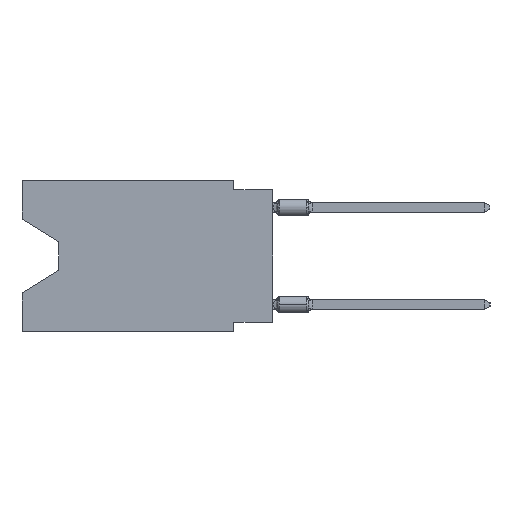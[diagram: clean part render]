
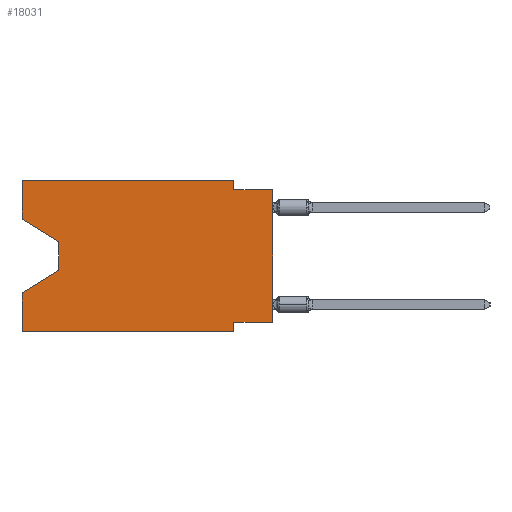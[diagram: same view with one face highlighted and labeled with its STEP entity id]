
A CAD part, left-side view. The second image highlights one B-rep face of the part: STEP entity #18031.
In plain terms, the highlighted planar face has unit normal (-1, 0, 0).
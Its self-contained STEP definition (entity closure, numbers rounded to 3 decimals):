
#53 = LINE ( 'NONE', #33759, #25097 ) ;
#741 = CARTESIAN_POINT ( 'NONE',  ( 0., 13.97, -5.893 ) ) ;
#848 = PLANE ( 'NONE',  #7714 ) ;
#1404 = EDGE_CURVE ( 'NONE', #9565, #9427, #14695, .T. ) ;
#1419 = VECTOR ( 'NONE', #7688, 1000. ) ;
#1522 = LINE ( 'NONE', #12523, #10236 ) ;
#2156 = CARTESIAN_POINT ( 'NONE',  ( 0., 16.383, -9.906 ) ) ;
#2433 = VECTOR ( 'NONE', #32776, 1000. ) ;
#2968 = VECTOR ( 'NONE', #32285, 1000. ) ;
#3423 = VERTEX_POINT ( 'NONE', #2156 ) ;
#4896 = VERTEX_POINT ( 'NONE', #17792 ) ;
#5262 = VECTOR ( 'NONE', #19988, 1000. ) ;
#5466 = CARTESIAN_POINT ( 'NONE',  ( 0., 2.54, -9.906 ) ) ;
#5565 = ORIENTED_EDGE ( 'NONE', *, *, #28004, .F. ) ;
#6286 = CARTESIAN_POINT ( 'NONE',  ( 0., 16.383, 0. ) ) ;
#6357 = ORIENTED_EDGE ( 'NONE', *, *, #11316, .T. ) ;
#6408 = VERTEX_POINT ( 'NONE', #21735 ) ;
#6618 = CARTESIAN_POINT ( 'NONE',  ( 0., 0., 0. ) ) ;
#6856 = VECTOR ( 'NONE', #31949, 1000. ) ;
#7027 = EDGE_CURVE ( 'NONE', #28562, #19460, #29848, .T. ) ;
#7688 = DIRECTION ( 'NONE',  ( 0., 0.855, -0.519 ) ) ;
#7714 = AXIS2_PLACEMENT_3D ( 'NONE', #21823, #32484, #32651 ) ;
#7912 = ORIENTED_EDGE ( 'NONE', *, *, #26705, .F. ) ;
#8039 = LINE ( 'NONE', #26431, #1419 ) ;
#8092 = EDGE_CURVE ( 'NONE', #6408, #10338, #29699, .T. ) ;
#8409 = FACE_OUTER_BOUND ( 'NONE', #16510, .T. ) ;
#8622 = CARTESIAN_POINT ( 'NONE',  ( 0., 16.383, 0. ) ) ;
#8834 = ORIENTED_EDGE ( 'NONE', *, *, #12111, .T. ) ;
#9427 = VERTEX_POINT ( 'NONE', #741 ) ;
#9565 = VERTEX_POINT ( 'NONE', #30663 ) ;
#9892 = CARTESIAN_POINT ( 'NONE',  ( 0., 16.383, -7.36 ) ) ;
#10169 = CARTESIAN_POINT ( 'NONE',  ( 0., 16.383, -9.906 ) ) ;
#10236 = VECTOR ( 'NONE', #30235, 1000. ) ;
#10338 = VERTEX_POINT ( 'NONE', #20717 ) ;
#10534 = DIRECTION ( 'NONE',  ( 0., 0., -1. ) ) ;
#11316 = EDGE_CURVE ( 'NONE', #3423, #22837, #25478, .T. ) ;
#11670 = ORIENTED_EDGE ( 'NONE', *, *, #33593, .F. ) ;
#12111 = EDGE_CURVE ( 'NONE', #16937, #10338, #19340, .T. ) ;
#12229 = ORIENTED_EDGE ( 'NONE', *, *, #7027, .F. ) ;
#12523 = CARTESIAN_POINT ( 'NONE',  ( 0., 16.383, 0. ) ) ;
#12594 = DIRECTION ( 'NONE',  ( 0., -1., 0. ) ) ;
#12970 = VECTOR ( 'NONE', #16502, 1000. ) ;
#13627 = DIRECTION ( 'NONE',  ( 0., 0., 1. ) ) ;
#14222 = LINE ( 'NONE', #29541, #2968 ) ;
#14631 = ORIENTED_EDGE ( 'NONE', *, *, #22446, .F. ) ;
#14695 = LINE ( 'NONE', #30330, #5262 ) ;
#15049 = VECTOR ( 'NONE', #12594, 1000. ) ;
#15448 = EDGE_CURVE ( 'NONE', #9427, #33056, #8039, .T. ) ;
#15841 = ORIENTED_EDGE ( 'NONE', *, *, #32622, .F. ) ;
#16502 = DIRECTION ( 'NONE',  ( 0., 1., 0. ) ) ;
#16510 = EDGE_LOOP ( 'NONE', ( #23887, #22128, #31767, #15841, #6357, #7912, #14631, #8834, #24074, #11670, #12229, #5565 ) ) ;
#16937 = VERTEX_POINT ( 'NONE', #25887 ) ;
#17792 = CARTESIAN_POINT ( 'NONE',  ( 0., 2.54, -9.271 ) ) ;
#18031 = ADVANCED_FACE ( 'NONE', ( #8409 ), #848, .F. ) ;
#18089 = VERTEX_POINT ( 'NONE', #29902 ) ;
#19340 = LINE ( 'NONE', #6618, #2433 ) ;
#19460 = VERTEX_POINT ( 'NONE', #20680 ) ;
#19988 = DIRECTION ( 'NONE',  ( 0., 0., -1. ) ) ;
#20680 = CARTESIAN_POINT ( 'NONE',  ( 0., 2.54, 0. ) ) ;
#20717 = CARTESIAN_POINT ( 'NONE',  ( 0., 0., -0.635 ) ) ;
#21065 = VECTOR ( 'NONE', #13627, 1000. ) ;
#21281 = CARTESIAN_POINT ( 'NONE',  ( 0., 0., -0.635 ) ) ;
#21349 = LINE ( 'NONE', #8622, #21065 ) ;
#21735 = CARTESIAN_POINT ( 'NONE',  ( 0., 2.54, -0.635 ) ) ;
#21823 = CARTESIAN_POINT ( 'NONE',  ( 0., 16.383, 0. ) ) ;
#22128 = ORIENTED_EDGE ( 'NONE', *, *, #1404, .T. ) ;
#22446 = EDGE_CURVE ( 'NONE', #16937, #4896, #31992, .T. ) ;
#22707 = DIRECTION ( 'NONE',  ( 0., 0., -1. ) ) ;
#22837 = VERTEX_POINT ( 'NONE', #5466 ) ;
#23887 = ORIENTED_EDGE ( 'NONE', *, *, #30106, .T. ) ;
#24074 = ORIENTED_EDGE ( 'NONE', *, *, #8092, .F. ) ;
#24728 = CARTESIAN_POINT ( 'NONE',  ( 0., 16.383, 0. ) ) ;
#25097 = VECTOR ( 'NONE', #10534, 1000. ) ;
#25478 = LINE ( 'NONE', #10169, #15049 ) ;
#25887 = CARTESIAN_POINT ( 'NONE',  ( 0., 0., -9.271 ) ) ;
#26077 = VECTOR ( 'NONE', #22707, 1000. ) ;
#26431 = CARTESIAN_POINT ( 'NONE',  ( 0., 13.97, -5.893 ) ) ;
#26705 = EDGE_CURVE ( 'NONE', #4896, #22837, #28432, .T. ) ;
#26842 = CARTESIAN_POINT ( 'NONE',  ( 0., 0., -9.271 ) ) ;
#27913 = CARTESIAN_POINT ( 'NONE',  ( 0., 2.54, -9.906 ) ) ;
#28004 = EDGE_CURVE ( 'NONE', #18089, #28562, #21349, .T. ) ;
#28432 = LINE ( 'NONE', #27913, #26077 ) ;
#28562 = VERTEX_POINT ( 'NONE', #24728 ) ;
#29541 = CARTESIAN_POINT ( 'NONE',  ( 0., 16.383, -2.546 ) ) ;
#29699 = LINE ( 'NONE', #21281, #6856 ) ;
#29848 = LINE ( 'NONE', #6286, #31558 ) ;
#29902 = CARTESIAN_POINT ( 'NONE',  ( 0., 16.383, -2.546 ) ) ;
#30106 = EDGE_CURVE ( 'NONE', #18089, #9565, #14222, .T. ) ;
#30235 = DIRECTION ( 'NONE',  ( 0., 0., 1. ) ) ;
#30330 = CARTESIAN_POINT ( 'NONE',  ( 0., 13.97, -4.013 ) ) ;
#30663 = CARTESIAN_POINT ( 'NONE',  ( 0., 13.97, -4.013 ) ) ;
#31558 = VECTOR ( 'NONE', #32600, 1000. ) ;
#31767 = ORIENTED_EDGE ( 'NONE', *, *, #15448, .T. ) ;
#31949 = DIRECTION ( 'NONE',  ( 0., -1., 0. ) ) ;
#31992 = LINE ( 'NONE', #26842, #12970 ) ;
#32285 = DIRECTION ( 'NONE',  ( 0., -0.855, -0.519 ) ) ;
#32484 = DIRECTION ( 'NONE',  ( 1., 0., 0. ) ) ;
#32600 = DIRECTION ( 'NONE',  ( 0., -1., 0. ) ) ;
#32622 = EDGE_CURVE ( 'NONE', #3423, #33056, #1522, .T. ) ;
#32651 = DIRECTION ( 'NONE',  ( 0., 0., -1. ) ) ;
#32776 = DIRECTION ( 'NONE',  ( 0., 0., 1. ) ) ;
#33056 = VERTEX_POINT ( 'NONE', #9892 ) ;
#33593 = EDGE_CURVE ( 'NONE', #19460, #6408, #53, .T. ) ;
#33759 = CARTESIAN_POINT ( 'NONE',  ( 0., 2.54, 0. ) ) ;
